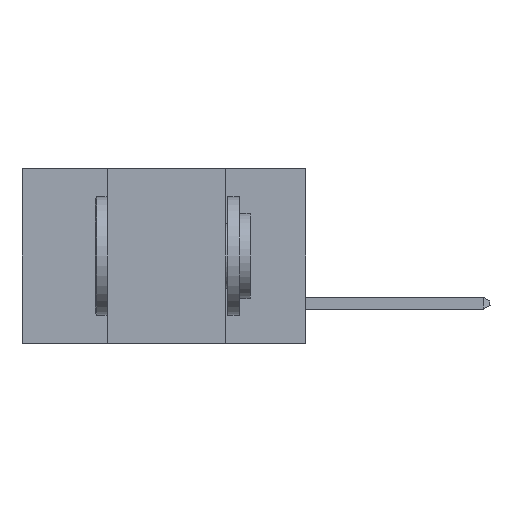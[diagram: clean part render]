
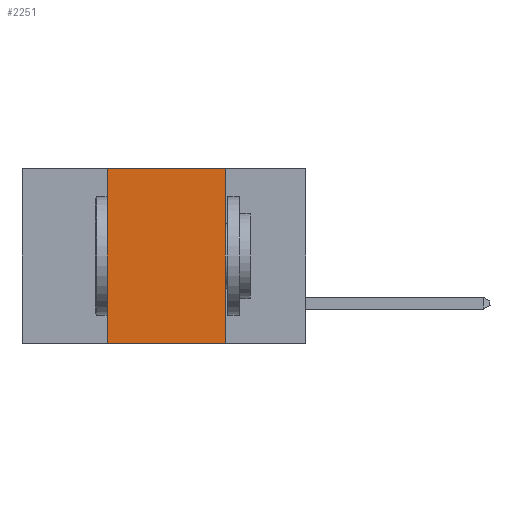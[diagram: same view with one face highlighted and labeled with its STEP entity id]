
A CAD part, left-side view. The second image highlights one B-rep face of the part: STEP entity #2251.
In plain terms, the highlighted planar face has unit normal (-1, 0, 0).
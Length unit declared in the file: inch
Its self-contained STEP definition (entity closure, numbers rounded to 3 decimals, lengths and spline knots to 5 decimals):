
#1163 = VERTEX_POINT ( 'NONE', #9872 ) ;
#1450 = ORIENTED_EDGE ( 'NONE', *, *, #2448, .F. ) ;
#2230 = LINE ( 'NONE', #20056, #27742 ) ;
#2251 = ADVANCED_FACE ( 'NONE', ( #25811 ), #28605, .F. ) ;
#2448 = EDGE_CURVE ( 'NONE', #5363, #1163, #26515, .T. ) ;
#4176 = ORIENTED_EDGE ( 'NONE', *, *, #24412, .T. ) ;
#4733 = VECTOR ( 'NONE', #6829, 39.37008 ) ;
#4814 = LINE ( 'NONE', #23702, #7356 ) ;
#5363 = VERTEX_POINT ( 'NONE', #29334 ) ;
#6829 = DIRECTION ( 'NONE',  ( 0., 0., -1. ) ) ;
#7356 = VECTOR ( 'NONE', #26064, 39.37008 ) ;
#7934 = CARTESIAN_POINT ( 'NONE',  ( 0., 0.6, 0. ) ) ;
#8028 = DIRECTION ( 'NONE',  ( 1., 0., 0. ) ) ;
#9262 = CARTESIAN_POINT ( 'NONE',  ( 0., 0.17, 0. ) ) ;
#9570 = EDGE_CURVE ( 'NONE', #26675, #5363, #2230, .T. ) ;
#9872 = CARTESIAN_POINT ( 'NONE',  ( 0., 0.17, 0. ) ) ;
#11669 = LINE ( 'NONE', #9262, #4733 ) ;
#13684 = EDGE_LOOP ( 'NONE', ( #22697, #1450, #15431, #4176 ) ) ;
#13991 = DIRECTION ( 'NONE',  ( 0., -1., 0. ) ) ;
#14384 = CARTESIAN_POINT ( 'NONE',  ( 0., 0.42, -0.37 ) ) ;
#15431 = ORIENTED_EDGE ( 'NONE', *, *, #9570, .F. ) ;
#16097 = CARTESIAN_POINT ( 'NONE',  ( 0., 0.6, 0. ) ) ;
#17889 = VERTEX_POINT ( 'NONE', #18208 ) ;
#18208 = CARTESIAN_POINT ( 'NONE',  ( 0., 0.17, -0.37 ) ) ;
#19953 = DIRECTION ( 'NONE',  ( 0., 0., 1. ) ) ;
#20056 = CARTESIAN_POINT ( 'NONE',  ( 0., 0.42, 0. ) ) ;
#21371 = AXIS2_PLACEMENT_3D ( 'NONE', #7934, #8028, #28905 ) ;
#22697 = ORIENTED_EDGE ( 'NONE', *, *, #27060, .F. ) ;
#23702 = CARTESIAN_POINT ( 'NONE',  ( 0., 0.6, -0.37 ) ) ;
#24412 = EDGE_CURVE ( 'NONE', #26675, #17889, #4814, .T. ) ;
#25779 = VECTOR ( 'NONE', #13991, 39.37008 ) ;
#25811 = FACE_OUTER_BOUND ( 'NONE', #13684, .T. ) ;
#26064 = DIRECTION ( 'NONE',  ( 0., -1., 0. ) ) ;
#26515 = LINE ( 'NONE', #16097, #25779 ) ;
#26675 = VERTEX_POINT ( 'NONE', #14384 ) ;
#27060 = EDGE_CURVE ( 'NONE', #1163, #17889, #11669, .T. ) ;
#27742 = VECTOR ( 'NONE', #19953, 39.37008 ) ;
#28605 = PLANE ( 'NONE',  #21371 ) ;
#28905 = DIRECTION ( 'NONE',  ( 0., 0., -1. ) ) ;
#29334 = CARTESIAN_POINT ( 'NONE',  ( 0., 0.42, 0. ) ) ;
